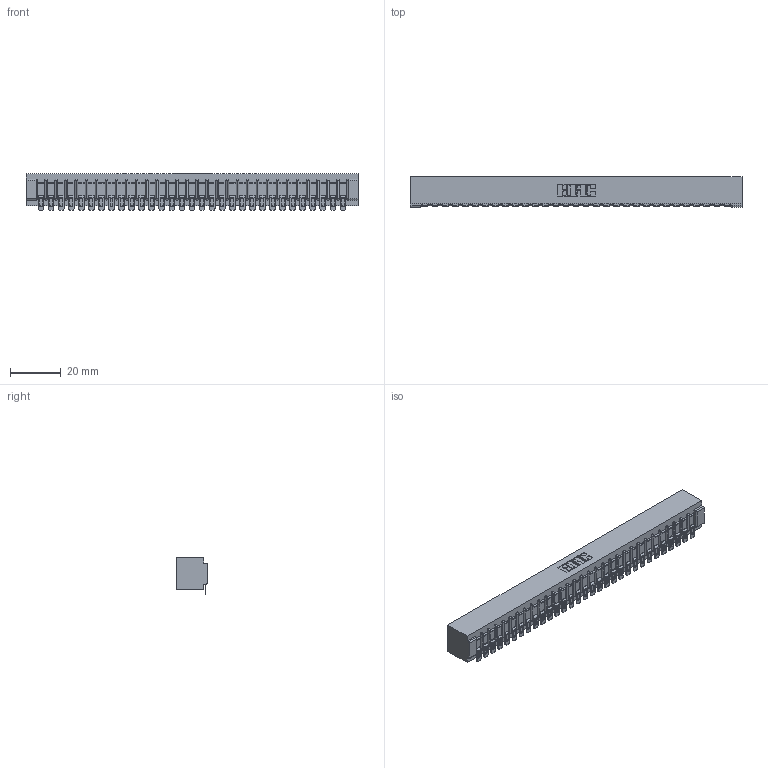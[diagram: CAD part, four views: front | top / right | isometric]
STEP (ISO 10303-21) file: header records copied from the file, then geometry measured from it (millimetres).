
FILE_DESCRIPTION (( 'STEP AP203' ), '1' );
FILE_NAME ('307-031-554-101.STEP', '2019-09-05T04:56:24', ( '' ), ( '' ), 'SwSTEP 2.0', 'SolidWorks 2016', '' );
FILE_SCHEMA (( 'CONFIG_CONTROL_DESIGN' ));
Length unit declared in the file: inch
Products named in the file (3): 307 Part_No Mounting Lugs; 307-290-002_554; 307-031-554-101
Assembly tree (32 placements, depth 2):
  307-031-554-101
    307 Part_No Mounting Lugs
    307-290-002_554  x31
Bounding box: 130.71 x 12.01 x 14.52 mm (x, y, z)
Volume: 14474.4 mm3; surface area: 18427.7 mm2
Topology: 32 solids, 32 shells, 2653 faces, 8142 edges, 5340 vertices
Faces by surface type: plane 1492, cylinder 1097, sphere 64
Entity records: 28619 total; most frequent: CARTESIAN_POINT 4826, ORIENTED_EDGE 4816, DIRECTION 4698, EDGE_CURVE 2408, VECTOR 1834, LINE 1834, VERTEX_POINT 1560, AXIS2_PLACEMENT_3D 1432
